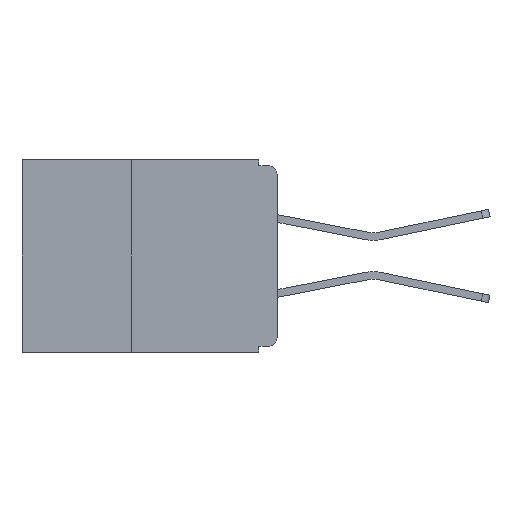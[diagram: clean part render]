
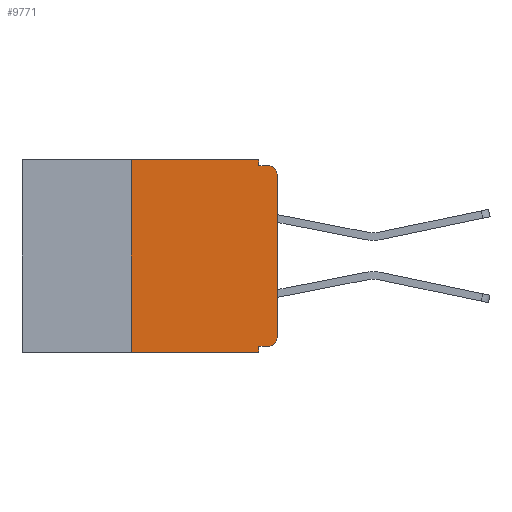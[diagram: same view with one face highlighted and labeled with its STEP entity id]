
A CAD part, left-side view. The second image highlights one B-rep face of the part: STEP entity #9771.
In plain terms, the highlighted planar face has unit normal (-1, 0, 0).
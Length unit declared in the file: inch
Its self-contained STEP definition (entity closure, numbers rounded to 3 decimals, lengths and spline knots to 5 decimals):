
#165 = ORIENTED_EDGE ( 'NONE', *, *, #28799, .F. ) ;
#229 = ORIENTED_EDGE ( 'NONE', *, *, #10119, .F. ) ;
#378 = ORIENTED_EDGE ( 'NONE', *, *, #22732, .F. ) ;
#422 = ORIENTED_EDGE ( 'NONE', *, *, #13246, .T. ) ;
#1503 = ORIENTED_EDGE ( 'NONE', *, *, #24617, .T. ) ;
#1523 = VERTEX_POINT ( 'NONE', #13130 ) ;
#2393 = VERTEX_POINT ( 'NONE', #33628 ) ;
#2750 = LINE ( 'NONE', #30881, #9094 ) ;
#3091 = CARTESIAN_POINT ( 'NONE',  ( 0., 0.031, -0.33 ) ) ;
#3234 = CARTESIAN_POINT ( 'NONE',  ( 0., 0.25, -0.33 ) ) ;
#3822 = CARTESIAN_POINT ( 'NONE',  ( 0., 0.25, 0. ) ) ;
#4194 = DIRECTION ( 'NONE',  ( 0., 0., 1. ) ) ;
#4332 = VERTEX_POINT ( 'NONE', #3091 ) ;
#5336 = CARTESIAN_POINT ( 'NONE',  ( 0., 0.031, -0.32 ) ) ;
#5606 = VECTOR ( 'NONE', #9011, 39.37008 ) ;
#6769 = ORIENTED_EDGE ( 'NONE', *, *, #33423, .F. ) ;
#7072 = CARTESIAN_POINT ( 'NONE',  ( 0., 0.015, -0.025 ) ) ;
#7551 = CIRCLE ( 'NONE', #19672, 0.015 ) ;
#7656 = CARTESIAN_POINT ( 'NONE',  ( 0., 0.031, -0.01 ) ) ;
#7883 = DIRECTION ( 'NONE',  ( -1., 0., 0. ) ) ;
#8105 = LINE ( 'NONE', #14661, #28181 ) ;
#9011 = DIRECTION ( 'NONE',  ( 0., -1., 0. ) ) ;
#9094 = VECTOR ( 'NONE', #28264, 39.37008 ) ;
#9771 = ADVANCED_FACE ( 'NONE', ( #13742 ), #24181, .F. ) ;
#9798 = DIRECTION ( 'NONE',  ( 0., 0., -1. ) ) ;
#10119 = EDGE_CURVE ( 'NONE', #1523, #27660, #2750, .T. ) ;
#10380 = ORIENTED_EDGE ( 'NONE', *, *, #12225, .F. ) ;
#10488 = LINE ( 'NONE', #3234, #22755 ) ;
#12225 = EDGE_CURVE ( 'NONE', #22044, #2393, #19693, .T. ) ;
#13130 = CARTESIAN_POINT ( 'NONE',  ( 0., 0.015, -0.32 ) ) ;
#13246 = EDGE_CURVE ( 'NONE', #1523, #13534, #17570, .T. ) ;
#13534 = VERTEX_POINT ( 'NONE', #22009 ) ;
#13661 = LINE ( 'NONE', #18248, #14461 ) ;
#13742 = FACE_OUTER_BOUND ( 'NONE', #19879, .T. ) ;
#13882 = DIRECTION ( 'NONE',  ( 1., 0., 0. ) ) ;
#14461 = VECTOR ( 'NONE', #33781, 39.37008 ) ;
#14661 = CARTESIAN_POINT ( 'NONE',  ( 0., 0.437, -0.33 ) ) ;
#15297 = ORIENTED_EDGE ( 'NONE', *, *, #29807, .F. ) ;
#15376 = VERTEX_POINT ( 'NONE', #15579 ) ;
#15579 = CARTESIAN_POINT ( 'NONE',  ( 0., 0.031, 0. ) ) ;
#15816 = EDGE_CURVE ( 'NONE', #13534, #16419, #28792, .T. ) ;
#16419 = VERTEX_POINT ( 'NONE', #22430 ) ;
#17283 = DIRECTION ( 'NONE',  ( 0., -1., 0. ) ) ;
#17483 = CARTESIAN_POINT ( 'NONE',  ( 0., 0., 0. ) ) ;
#17570 = CIRCLE ( 'NONE', #19064, 0.015 ) ;
#18007 = CARTESIAN_POINT ( 'NONE',  ( 0., 0.25, -0.33 ) ) ;
#18248 = CARTESIAN_POINT ( 'NONE',  ( 0., 0.437, 0. ) ) ;
#18664 = VERTEX_POINT ( 'NONE', #18007 ) ;
#19064 = AXIS2_PLACEMENT_3D ( 'NONE', #23611, #7883, #26249 ) ;
#19171 = VECTOR ( 'NONE', #19906, 39.37008 ) ;
#19672 = AXIS2_PLACEMENT_3D ( 'NONE', #7072, #25444, #9798 ) ;
#19693 = LINE ( 'NONE', #27319, #5606 ) ;
#19879 = EDGE_LOOP ( 'NONE', ( #25546, #25964, #10380, #6769, #378, #15297, #1503, #165, #229, #422 ) ) ;
#19906 = DIRECTION ( 'NONE',  ( 0., 0., -1. ) ) ;
#20105 = EDGE_CURVE ( 'NONE', #16419, #2393, #7551, .T. ) ;
#21081 = VECTOR ( 'NONE', #4194, 39.37008 ) ;
#22009 = CARTESIAN_POINT ( 'NONE',  ( 0., 0., -0.305 ) ) ;
#22044 = VERTEX_POINT ( 'NONE', #7656 ) ;
#22066 = VECTOR ( 'NONE', #31421, 39.37008 ) ;
#22430 = CARTESIAN_POINT ( 'NONE',  ( 0., 0., -0.025 ) ) ;
#22521 = CARTESIAN_POINT ( 'NONE',  ( 0., 0.031, -0.33 ) ) ;
#22732 = EDGE_CURVE ( 'NONE', #25271, #15376, #13661, .T. ) ;
#22755 = VECTOR ( 'NONE', #29615, 39.37008 ) ;
#23611 = CARTESIAN_POINT ( 'NONE',  ( 0., 0.015, -0.305 ) ) ;
#24181 = PLANE ( 'NONE',  #32060 ) ;
#24617 = EDGE_CURVE ( 'NONE', #18664, #4332, #8105, .T. ) ;
#25271 = VERTEX_POINT ( 'NONE', #3822 ) ;
#25444 = DIRECTION ( 'NONE',  ( -1., 0., 0. ) ) ;
#25546 = ORIENTED_EDGE ( 'NONE', *, *, #15816, .T. ) ;
#25964 = ORIENTED_EDGE ( 'NONE', *, *, #20105, .T. ) ;
#26249 = DIRECTION ( 'NONE',  ( 0., 0., -1. ) ) ;
#27319 = CARTESIAN_POINT ( 'NONE',  ( 0., 0., -0.01 ) ) ;
#27660 = VERTEX_POINT ( 'NONE', #5336 ) ;
#28181 = VECTOR ( 'NONE', #17283, 39.37008 ) ;
#28264 = DIRECTION ( 'NONE',  ( 0., 1., 0. ) ) ;
#28790 = CARTESIAN_POINT ( 'NONE',  ( 0., 0.031, 0. ) ) ;
#28792 = LINE ( 'NONE', #17483, #21081 ) ;
#28799 = EDGE_CURVE ( 'NONE', #27660, #4332, #32984, .T. ) ;
#29419 = CARTESIAN_POINT ( 'NONE',  ( 0., 0.437, 0. ) ) ;
#29615 = DIRECTION ( 'NONE',  ( 0., 0., 1. ) ) ;
#29801 = LINE ( 'NONE', #28790, #22066 ) ;
#29807 = EDGE_CURVE ( 'NONE', #18664, #25271, #10488, .T. ) ;
#30881 = CARTESIAN_POINT ( 'NONE',  ( 0., 0., -0.32 ) ) ;
#31421 = DIRECTION ( 'NONE',  ( 0., 0., -1. ) ) ;
#32044 = DIRECTION ( 'NONE',  ( 0., 0., -1. ) ) ;
#32060 = AXIS2_PLACEMENT_3D ( 'NONE', #29419, #13882, #32044 ) ;
#32984 = LINE ( 'NONE', #22521, #19171 ) ;
#33423 = EDGE_CURVE ( 'NONE', #15376, #22044, #29801, .T. ) ;
#33628 = CARTESIAN_POINT ( 'NONE',  ( 0., 0.015, -0.01 ) ) ;
#33781 = DIRECTION ( 'NONE',  ( 0., -1., 0. ) ) ;
